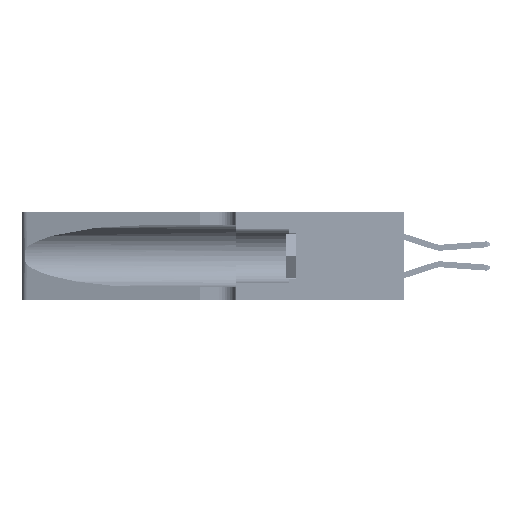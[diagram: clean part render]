
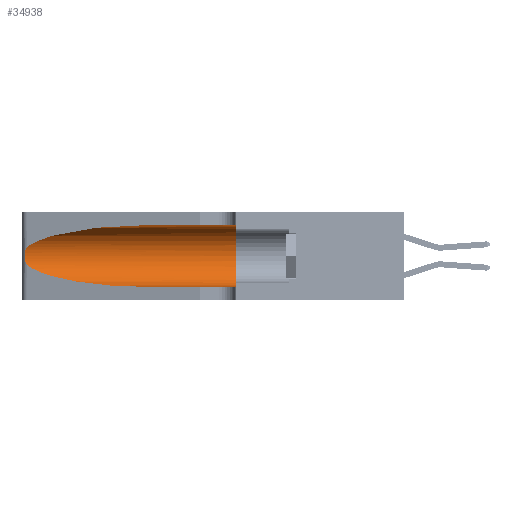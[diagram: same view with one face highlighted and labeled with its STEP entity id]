
A CAD part, left-side view. The second image highlights one B-rep face of the part: STEP entity #34938.
In plain terms, the highlighted cylindrical face has radius 3.308 mm (diameter 6.617 mm), a partial arc.
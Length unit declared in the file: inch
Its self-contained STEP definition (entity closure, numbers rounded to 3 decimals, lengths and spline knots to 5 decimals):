
#479 = VERTEX_POINT ( 'NONE', #32457 ) ;
#1745 = AXIS2_PLACEMENT_3D ( 'NONE', #36062, #32106, #25050 ) ;
#4248 = CARTESIAN_POINT ( 'NONE',  ( 0.1305, 0.72297, 0.31525 ) ) ;
#4372 = EDGE_CURVE ( 'NONE', #43315, #16467, #26439, .T. ) ;
#6114 = LINE ( 'NONE', #15581, #34162 ) ;
#6739 = AXIS2_PLACEMENT_3D ( 'NONE', #29347, #36592, #15097 ) ;
#7395 = CYLINDRICAL_SURFACE ( 'NONE', #6739, 0.13025 ) ;
#9422 = CARTESIAN_POINT ( 'NONE',  ( 0.18966, 0.96281, 0.31525 ) ) ;
#11143 = CARTESIAN_POINT ( 'NONE',  ( 0.25639, 1.23186, 0.15144 ) ) ;
#11299 = CARTESIAN_POINT ( 'NONE',  ( 0.26075, 1.23896, 0.19203 ) ) ;
#11433 = CARTESIAN_POINT ( 'NONE',  ( 0.25487, 1.22718, 0.14631 ) ) ;
#11526 = CARTESIAN_POINT ( 'NONE',  ( 0.1305, 0.72297, 0.05475 ) ) ;
#11678 = CARTESIAN_POINT ( 'NONE',  ( 0.18966, 0.96281, 0.05475 ) ) ;
#12299 = CIRCLE ( 'NONE', #1745, 0.13025 ) ;
#13167 = ORIENTED_EDGE ( 'NONE', *, *, #16286, .F. ) ;
#14584 = CARTESIAN_POINT ( 'NONE',  ( 0.25856, 1.23593, 0.16098 ) ) ;
#15097 = DIRECTION ( 'NONE',  ( 0., 0., -1. ) ) ;
#15581 = CARTESIAN_POINT ( 'NONE',  ( 0.1305, 1.61858, 0.31525 ) ) ;
#16286 = EDGE_CURVE ( 'NONE', #479, #31944, #12299, .T. ) ;
#16467 = VERTEX_POINT ( 'NONE', #11433 ) ;
#16584 = VERTEX_POINT ( 'NONE', #23032 ) ;
#16636 = ORIENTED_EDGE ( 'NONE', *, *, #41946, .T. ) ;
#19647 = CARTESIAN_POINT ( 'NONE',  ( 0.25487, 1.22718, 0.22369 ) ) ;
#21074 = EDGE_LOOP ( 'NONE', ( #22837, #33214, #16636, #34141, #13167, #38114 ) ) ;
#21642 = CARTESIAN_POINT ( 'NONE',  ( 0.25555, 1.22994, 0.2215 ) ) ;
#22837 = ORIENTED_EDGE ( 'NONE', *, *, #39600, .T. ) ;
#23032 = CARTESIAN_POINT ( 'NONE',  ( 0.1305, 0.72297, 0.05475 ) ) ;
#25050 = DIRECTION ( 'NONE',  ( 0., 0., 1. ) ) ;
#25220 = CARTESIAN_POINT ( 'NONE',  ( 0.25487, 1.22718, 0.14631 ) ) ;
#25372 = CARTESIAN_POINT ( 'NONE',  ( 0.25555, 1.22993, 0.14849 ) ) ;
#25599 = CARTESIAN_POINT ( 'NONE',  ( 0.2373, 1.15595, 0.08982 ) ) ;
#26234 = EDGE_CURVE ( 'NONE', #35624, #479, #6114, .T. ) ;
#26439 = B_SPLINE_CURVE_WITH_KNOTS ( 'NONE', 3,
 ( #32753, #21642, #39857, #43451, #32606, #36233, #11299, #36073, #28691, #14584, #36391, #11143, #25372, #25220 ),
 .UNSPECIFIED., .F., .F.,
 ( 4, 2, 2, 2, 2, 2, 4 ),
 ( 0., 0.00027, 0.00053, 0.00107, 0.0016, 0.00187, 0.00214 ),
 .UNSPECIFIED. ) ;
#27557 = FACE_OUTER_BOUND ( 'NONE', #21074, .T. ) ;
#27569 = DIRECTION ( 'NONE',  ( 0., -1., 0. ) ) ;
#28691 = CARTESIAN_POINT ( 'NONE',  ( 0.26017, 1.23833, 0.17102 ) ) ;
#29347 = CARTESIAN_POINT ( 'NONE',  ( 0.1305, 1.61858, 0.185 ) ) ;
#31583 = VECTOR ( 'NONE', #27569, 39.37008 ) ;
#31944 = VERTEX_POINT ( 'NONE', #39524 ) ;
#32106 = DIRECTION ( 'NONE',  ( 0., 1., 0. ) ) ;
#32457 = CARTESIAN_POINT ( 'NONE',  ( 0.1305, 0.35, 0.31525 ) ) ;
#32606 = CARTESIAN_POINT ( 'NONE',  ( 0.25854, 1.2359, 0.20912 ) ) ;
#32753 = CARTESIAN_POINT ( 'NONE',  ( 0.25487, 1.22718, 0.22369 ) ) ;
#33145 = CARTESIAN_POINT ( 'NONE',  ( 0.25487, 1.22718, 0.14631 ) ) ;
#33214 = ORIENTED_EDGE ( 'NONE', *, *, #4372, .T. ) ;
#33436 = DIRECTION ( 'NONE',  ( 0., -1., 0. ) ) ;
#33763 = EDGE_CURVE ( 'NONE', #16584, #31944, #44545, .T. ) ;
#34141 = ORIENTED_EDGE ( 'NONE', *, *, #33763, .T. ) ;
#34162 = VECTOR ( 'NONE', #33436, 39.37008 ) ;
#34938 = ADVANCED_FACE ( 'NONE', ( #27557 ), #7395, .F. ) ;
#35624 = VERTEX_POINT ( 'NONE', #4248 ) ;
#36062 = CARTESIAN_POINT ( 'NONE',  ( 0.1305, 0.35, 0.185 ) ) ;
#36073 = CARTESIAN_POINT ( 'NONE',  ( 0.26075, 1.23896, 0.178 ) ) ;
#36233 = CARTESIAN_POINT ( 'NONE',  ( 0.26018, 1.23835, 0.19895 ) ) ;
#36391 = CARTESIAN_POINT ( 'NONE',  ( 0.25789, 1.23486, 0.15765 ) ) ;
#36592 = DIRECTION ( 'NONE',  ( 0., -1., 0. ) ) ;
#38114 = ORIENTED_EDGE ( 'NONE', *, *, #26234, .F. ) ;
#38250 =( BOUNDED_CURVE ( )  B_SPLINE_CURVE ( 3, ( #33145, #25599, #11678, #11526 ),
 .UNSPECIFIED., .F., .F. ) 
 B_SPLINE_CURVE_WITH_KNOTS ( ( 4, 4 ),
 ( 3.44316, 4.71239 ),
 .UNSPECIFIED. ) 
 CURVE ( )  GEOMETRIC_REPRESENTATION_ITEM ( )  RATIONAL_B_SPLINE_CURVE ( ( 1., 0.87, 0.87, 1. ) ) 
 REPRESENTATION_ITEM ( '' )  );
#38581 = CARTESIAN_POINT ( 'NONE',  ( 0.1305, 1.61858, 0.05475 ) ) ;
#39524 = CARTESIAN_POINT ( 'NONE',  ( 0.1305, 0.35, 0.05475 ) ) ;
#39600 = EDGE_CURVE ( 'NONE', #35624, #43315, #43984, .T. ) ;
#39857 = CARTESIAN_POINT ( 'NONE',  ( 0.25639, 1.23184, 0.21858 ) ) ;
#41143 = CARTESIAN_POINT ( 'NONE',  ( 0.1305, 0.72297, 0.31525 ) ) ;
#41946 = EDGE_CURVE ( 'NONE', #16467, #16584, #38250, .T. ) ;
#43315 = VERTEX_POINT ( 'NONE', #44210 ) ;
#43451 = CARTESIAN_POINT ( 'NONE',  ( 0.25787, 1.23484, 0.2124 ) ) ;
#43984 =( BOUNDED_CURVE ( )  B_SPLINE_CURVE ( 3, ( #41143, #9422, #44560, #19647 ),
 .UNSPECIFIED., .F., .T. ) 
 B_SPLINE_CURVE_WITH_KNOTS ( ( 4, 4 ),
 ( 1.5708, 2.84003 ),
 .UNSPECIFIED. ) 
 CURVE ( )  GEOMETRIC_REPRESENTATION_ITEM ( )  RATIONAL_B_SPLINE_CURVE ( ( 1., 0.87, 0.87, 1. ) ) 
 REPRESENTATION_ITEM ( '' )  );
#44210 = CARTESIAN_POINT ( 'NONE',  ( 0.25487, 1.22718, 0.22369 ) ) ;
#44545 = LINE ( 'NONE', #38581, #31583 ) ;
#44560 = CARTESIAN_POINT ( 'NONE',  ( 0.2373, 1.15595, 0.28018 ) ) ;
